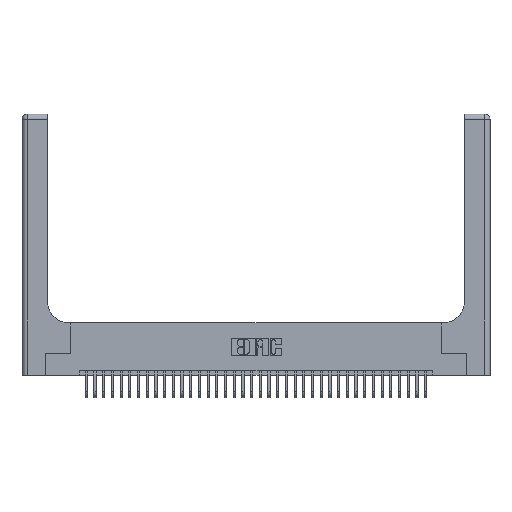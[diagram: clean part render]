
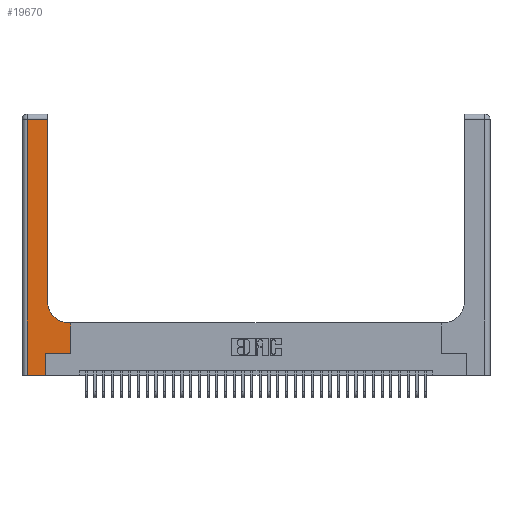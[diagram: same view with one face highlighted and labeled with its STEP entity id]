
A CAD part, top view. The second image highlights one B-rep face of the part: STEP entity #19670.
In plain terms, the highlighted planar face has unit normal (0, 0, 1).
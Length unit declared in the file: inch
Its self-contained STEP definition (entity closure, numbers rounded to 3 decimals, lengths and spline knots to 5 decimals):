
#31 = VERTEX_POINT ( 'NONE', #3526 ) ;
#195 = EDGE_CURVE ( 'NONE', #3372, #32814, #9145, .T. ) ;
#226 = CARTESIAN_POINT ( 'NONE',  ( 0.5415, 0.85, 0.37 ) ) ;
#474 = EDGE_CURVE ( 'NONE', #31, #3372, #37455, .T. ) ;
#722 = ORIENTED_EDGE ( 'NONE', *, *, #25548, .T. ) ;
#1022 = CARTESIAN_POINT ( 'NONE',  ( 0., 3., 0.37 ) ) ;
#1164 = VECTOR ( 'NONE', #19339, 39.37008 ) ;
#1721 = LINE ( 'NONE', #1779, #2671 ) ;
#1779 = CARTESIAN_POINT ( 'NONE',  ( 0.269, 0., 0.37 ) ) ;
#2260 = CARTESIAN_POINT ( 'NONE',  ( 0.2915, 3., 0.37 ) ) ;
#2529 = AXIS2_PLACEMENT_3D ( 'NONE', #226, #21123, #3220 ) ;
#2635 = CARTESIAN_POINT ( 'NONE',  ( 0., 0., 0.37 ) ) ;
#2671 = VECTOR ( 'NONE', #4794, 39.37008 ) ;
#3106 = EDGE_CURVE ( 'NONE', #17765, #20592, #5162, .T. ) ;
#3220 = DIRECTION ( 'NONE',  ( 1., 0., 0. ) ) ;
#3372 = VERTEX_POINT ( 'NONE', #24919 ) ;
#3392 = VERTEX_POINT ( 'NONE', #4037 ) ;
#3526 = CARTESIAN_POINT ( 'NONE',  ( 0.5585, 0.25, 0.37 ) ) ;
#3894 = EDGE_CURVE ( 'NONE', #32814, #26273, #10747, .T. ) ;
#3902 = VECTOR ( 'NONE', #26118, 39.37008 ) ;
#4037 = CARTESIAN_POINT ( 'NONE',  ( 0.269, 0.25, 0.37 ) ) ;
#4794 = DIRECTION ( 'NONE',  ( 0., 1., 0. ) ) ;
#5162 = LINE ( 'NONE', #2635, #35855 ) ;
#5733 = DIRECTION ( 'NONE',  ( 0., 1., 0. ) ) ;
#5985 = ORIENTED_EDGE ( 'NONE', *, *, #20327, .T. ) ;
#6772 = VECTOR ( 'NONE', #22172, 39.37008 ) ;
#7057 = PLANE ( 'NONE',  #32308 ) ;
#7778 = DIRECTION ( 'NONE',  ( -1., 0., 0. ) ) ;
#9145 = LINE ( 'NONE', #13369, #1164 ) ;
#9618 = ORIENTED_EDGE ( 'NONE', *, *, #3106, .T. ) ;
#9900 = CARTESIAN_POINT ( 'NONE',  ( 0.269, 0.25, 0.37 ) ) ;
#10079 = DIRECTION ( 'NONE',  ( 0., 0., -1. ) ) ;
#10747 = CIRCLE ( 'NONE', #2529, 0.25 ) ;
#11350 = EDGE_CURVE ( 'NONE', #36085, #17765, #30506, .T. ) ;
#12853 = VERTEX_POINT ( 'NONE', #27628 ) ;
#12920 = DIRECTION ( 'NONE',  ( 1., 0., 0. ) ) ;
#13369 = CARTESIAN_POINT ( 'NONE',  ( 0.2915, 0.6, 0.37 ) ) ;
#15097 = ORIENTED_EDGE ( 'NONE', *, *, #11350, .T. ) ;
#15729 = CARTESIAN_POINT ( 'NONE',  ( 0.2915, 0.85, 0.37 ) ) ;
#16399 = VECTOR ( 'NONE', #7778, 39.37008 ) ;
#17765 = VERTEX_POINT ( 'NONE', #33997 ) ;
#18299 = LINE ( 'NONE', #9900, #33138 ) ;
#19339 = DIRECTION ( 'NONE',  ( -1., 0., 0. ) ) ;
#19670 = ADVANCED_FACE ( 'NONE', ( #31795 ), #7057, .F. ) ;
#19812 = LINE ( 'NONE', #2260, #3902 ) ;
#20327 = EDGE_CURVE ( 'NONE', #3392, #31, #18299, .T. ) ;
#20592 = VERTEX_POINT ( 'NONE', #23051 ) ;
#21123 = DIRECTION ( 'NONE',  ( 0., 0., -1. ) ) ;
#21715 = VECTOR ( 'NONE', #5733, 39.37008 ) ;
#22172 = DIRECTION ( 'NONE',  ( 0., -1., 0. ) ) ;
#22683 = CARTESIAN_POINT ( 'NONE',  ( 0.5415, 0.6, 0.37 ) ) ;
#22890 = EDGE_CURVE ( 'NONE', #20592, #3392, #1721, .T. ) ;
#23051 = CARTESIAN_POINT ( 'NONE',  ( 0.269, 0., 0.37 ) ) ;
#24303 = LINE ( 'NONE', #34415, #16399 ) ;
#24919 = CARTESIAN_POINT ( 'NONE',  ( 0.5585, 0.6, 0.37 ) ) ;
#25407 = ORIENTED_EDGE ( 'NONE', *, *, #195, .T. ) ;
#25548 = EDGE_CURVE ( 'NONE', #26273, #12853, #19812, .T. ) ;
#26118 = DIRECTION ( 'NONE',  ( 0., 1., 0. ) ) ;
#26273 = VERTEX_POINT ( 'NONE', #15729 ) ;
#27628 = CARTESIAN_POINT ( 'NONE',  ( 0.2915, 2.94, 0.37 ) ) ;
#27999 = CARTESIAN_POINT ( 'NONE',  ( 0.06, 3., 0.37 ) ) ;
#30300 = ORIENTED_EDGE ( 'NONE', *, *, #474, .T. ) ;
#30506 = LINE ( 'NONE', #27999, #6772 ) ;
#30854 = DIRECTION ( 'NONE',  ( -1., 0., 0. ) ) ;
#31669 = CARTESIAN_POINT ( 'NONE',  ( 0.06, 2.94, 0.37 ) ) ;
#31795 = FACE_OUTER_BOUND ( 'NONE', #37684, .T. ) ;
#32308 = AXIS2_PLACEMENT_3D ( 'NONE', #1022, #10079, #30854 ) ;
#32402 = CARTESIAN_POINT ( 'NONE',  ( 0.5585, 0.25, 0.37 ) ) ;
#32573 = ORIENTED_EDGE ( 'NONE', *, *, #33387, .T. ) ;
#32814 = VERTEX_POINT ( 'NONE', #22683 ) ;
#33138 = VECTOR ( 'NONE', #12920, 39.37008 ) ;
#33387 = EDGE_CURVE ( 'NONE', #12853, #36085, #24303, .T. ) ;
#33997 = CARTESIAN_POINT ( 'NONE',  ( 0.06, 0., 0.37 ) ) ;
#34415 = CARTESIAN_POINT ( 'NONE',  ( 0., 2.94, 0.37 ) ) ;
#35544 = DIRECTION ( 'NONE',  ( 1., 0., 0. ) ) ;
#35855 = VECTOR ( 'NONE', #35544, 39.37008 ) ;
#36085 = VERTEX_POINT ( 'NONE', #31669 ) ;
#36508 = ORIENTED_EDGE ( 'NONE', *, *, #3894, .T. ) ;
#37455 = LINE ( 'NONE', #32402, #21715 ) ;
#37684 = EDGE_LOOP ( 'NONE', ( #722, #32573, #15097, #9618, #38340, #5985, #30300, #25407, #36508 ) ) ;
#38340 = ORIENTED_EDGE ( 'NONE', *, *, #22890, .T. ) ;
